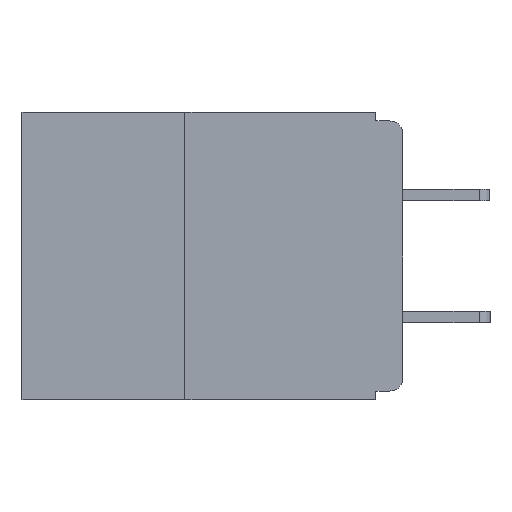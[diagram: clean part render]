
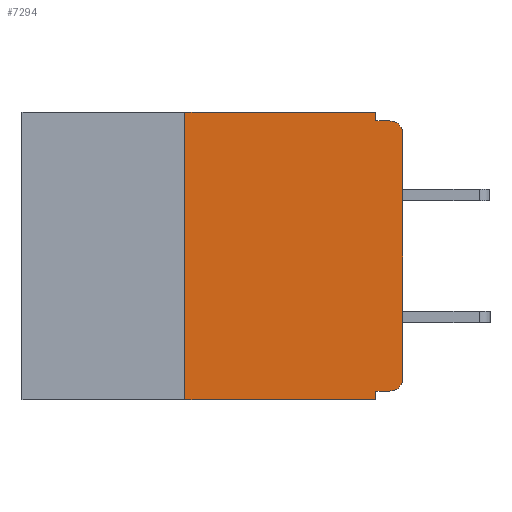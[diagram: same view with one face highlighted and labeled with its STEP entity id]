
A CAD part, left-side view. The second image highlights one B-rep face of the part: STEP entity #7294.
In plain terms, the highlighted planar face has unit normal (-1, 0, 0).
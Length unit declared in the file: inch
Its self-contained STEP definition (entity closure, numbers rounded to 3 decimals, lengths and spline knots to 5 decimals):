
#58 = VECTOR ( 'NONE', #5269, 39.37008 ) ;
#281 = CIRCLE ( 'NONE', #8449, 0.015 ) ;
#444 = EDGE_CURVE ( 'NONE', #9621, #3696, #555, .T. ) ;
#460 = DIRECTION ( 'NONE',  ( 0., -1., 0. ) ) ;
#555 = LINE ( 'NONE', #4936, #4952 ) ;
#560 = EDGE_CURVE ( 'NONE', #3987, #4251, #6206, .T. ) ;
#705 = DIRECTION ( 'NONE',  ( 0., 0., 1. ) ) ;
#847 = AXIS2_PLACEMENT_3D ( 'NONE', #3972, #2289, #8373 ) ;
#866 = EDGE_CURVE ( 'NONE', #9621, #1236, #281, .T. ) ;
#1070 = CARTESIAN_POINT ( 'NONE',  ( 0., 0.015, -0.025 ) ) ;
#1236 = VERTEX_POINT ( 'NONE', #2283 ) ;
#1337 = DIRECTION ( 'NONE',  ( -1., 0., 0. ) ) ;
#1426 = PLANE ( 'NONE',  #847 ) ;
#1719 = VECTOR ( 'NONE', #6073, 39.37008 ) ;
#1726 = EDGE_CURVE ( 'NONE', #8494, #4510, #2297, .T. ) ;
#1807 = CARTESIAN_POINT ( 'NONE',  ( 0., 0.031, -0.01 ) ) ;
#1955 = VERTEX_POINT ( 'NONE', #3470 ) ;
#2042 = VECTOR ( 'NONE', #6081, 39.37008 ) ;
#2283 = CARTESIAN_POINT ( 'NONE',  ( 0., 0., -0.305 ) ) ;
#2289 = DIRECTION ( 'NONE',  ( 1., 0., 0. ) ) ;
#2297 = LINE ( 'NONE', #6161, #2042 ) ;
#2513 = VECTOR ( 'NONE', #6320, 39.37008 ) ;
#2748 = FACE_OUTER_BOUND ( 'NONE', #8184, .T. ) ;
#2937 = LINE ( 'NONE', #3355, #5014 ) ;
#2980 = EDGE_CURVE ( 'NONE', #1236, #3987, #2937, .T. ) ;
#3061 = VECTOR ( 'NONE', #460, 39.37008 ) ;
#3185 = VECTOR ( 'NONE', #5602, 39.37008 ) ;
#3286 = VERTEX_POINT ( 'NONE', #1807 ) ;
#3355 = CARTESIAN_POINT ( 'NONE',  ( 0., 0., 0. ) ) ;
#3467 = AXIS2_PLACEMENT_3D ( 'NONE', #1070, #1337, #10816 ) ;
#3470 = CARTESIAN_POINT ( 'NONE',  ( 0., 0.031, -0.33 ) ) ;
#3534 = EDGE_CURVE ( 'NONE', #3286, #4251, #10138, .T. ) ;
#3696 = VERTEX_POINT ( 'NONE', #10712 ) ;
#3972 = CARTESIAN_POINT ( 'NONE',  ( 0., 0.437, 0. ) ) ;
#3987 = VERTEX_POINT ( 'NONE', #4921 ) ;
#4251 = VERTEX_POINT ( 'NONE', #10725 ) ;
#4510 = VERTEX_POINT ( 'NONE', #7284 ) ;
#4891 = VERTEX_POINT ( 'NONE', #6075 ) ;
#4921 = CARTESIAN_POINT ( 'NONE',  ( 0., 0., -0.025 ) ) ;
#4936 = CARTESIAN_POINT ( 'NONE',  ( 0., 0., -0.32 ) ) ;
#4952 = VECTOR ( 'NONE', #6053, 39.37008 ) ;
#5014 = VECTOR ( 'NONE', #705, 39.37008 ) ;
#5214 = CARTESIAN_POINT ( 'NONE',  ( 0., 0.031, -0.33 ) ) ;
#5269 = DIRECTION ( 'NONE',  ( 0., 0., -1. ) ) ;
#5558 = LINE ( 'NONE', #5728, #3185 ) ;
#5602 = DIRECTION ( 'NONE',  ( 0., -1., 0. ) ) ;
#5677 = EDGE_CURVE ( 'NONE', #4510, #3286, #6668, .T. ) ;
#5723 = EDGE_CURVE ( 'NONE', #4891, #8494, #10717, .T. ) ;
#5728 = CARTESIAN_POINT ( 'NONE',  ( 0., 0.437, -0.33 ) ) ;
#5731 = ORIENTED_EDGE ( 'NONE', *, *, #2980, .T. ) ;
#5779 = EDGE_CURVE ( 'NONE', #4891, #1955, #5558, .T. ) ;
#5855 = EDGE_CURVE ( 'NONE', #3696, #1955, #9276, .T. ) ;
#5886 = ORIENTED_EDGE ( 'NONE', *, *, #560, .T. ) ;
#6024 = ORIENTED_EDGE ( 'NONE', *, *, #3534, .F. ) ;
#6045 = ORIENTED_EDGE ( 'NONE', *, *, #5677, .F. ) ;
#6053 = DIRECTION ( 'NONE',  ( 0., 1., 0. ) ) ;
#6073 = DIRECTION ( 'NONE',  ( 0., 0., 1. ) ) ;
#6075 = CARTESIAN_POINT ( 'NONE',  ( 0., 0.25, -0.33 ) ) ;
#6081 = DIRECTION ( 'NONE',  ( 0., -1., 0. ) ) ;
#6116 = ORIENTED_EDGE ( 'NONE', *, *, #1726, .F. ) ;
#6129 = ORIENTED_EDGE ( 'NONE', *, *, #5723, .F. ) ;
#6161 = CARTESIAN_POINT ( 'NONE',  ( 0., 0.437, 0. ) ) ;
#6206 = CIRCLE ( 'NONE', #3467, 0.015 ) ;
#6246 = CARTESIAN_POINT ( 'NONE',  ( 0., 0.25, -0.33 ) ) ;
#6293 = ORIENTED_EDGE ( 'NONE', *, *, #5779, .T. ) ;
#6320 = DIRECTION ( 'NONE',  ( 0., 0., -1. ) ) ;
#6411 = CARTESIAN_POINT ( 'NONE',  ( 0., 0.031, 0. ) ) ;
#6457 = ORIENTED_EDGE ( 'NONE', *, *, #5855, .F. ) ;
#6560 = ORIENTED_EDGE ( 'NONE', *, *, #444, .F. ) ;
#6668 = LINE ( 'NONE', #6411, #2513 ) ;
#6788 = ORIENTED_EDGE ( 'NONE', *, *, #866, .T. ) ;
#7102 = DIRECTION ( 'NONE',  ( -1., 0., 0. ) ) ;
#7141 = CARTESIAN_POINT ( 'NONE',  ( 0., 0.015, -0.305 ) ) ;
#7284 = CARTESIAN_POINT ( 'NONE',  ( 0., 0.031, 0. ) ) ;
#7294 = ADVANCED_FACE ( 'NONE', ( #2748 ), #1426, .F. ) ;
#7369 = DIRECTION ( 'NONE',  ( 0., 0., -1. ) ) ;
#7483 = CARTESIAN_POINT ( 'NONE',  ( 0., 0.25, 0. ) ) ;
#8184 = EDGE_LOOP ( 'NONE', ( #5731, #5886, #6024, #6045, #6116, #6129, #6293, #6457, #6560, #6788 ) ) ;
#8373 = DIRECTION ( 'NONE',  ( 0., 0., -1. ) ) ;
#8449 = AXIS2_PLACEMENT_3D ( 'NONE', #7141, #7102, #7369 ) ;
#8494 = VERTEX_POINT ( 'NONE', #7483 ) ;
#9276 = LINE ( 'NONE', #5214, #58 ) ;
#9621 = VERTEX_POINT ( 'NONE', #10536 ) ;
#10138 = LINE ( 'NONE', #10289, #3061 ) ;
#10289 = CARTESIAN_POINT ( 'NONE',  ( 0., 0., -0.01 ) ) ;
#10536 = CARTESIAN_POINT ( 'NONE',  ( 0., 0.015, -0.32 ) ) ;
#10712 = CARTESIAN_POINT ( 'NONE',  ( 0., 0.031, -0.32 ) ) ;
#10717 = LINE ( 'NONE', #6246, #1719 ) ;
#10725 = CARTESIAN_POINT ( 'NONE',  ( 0., 0.015, -0.01 ) ) ;
#10816 = DIRECTION ( 'NONE',  ( 0., 0., -1. ) ) ;
